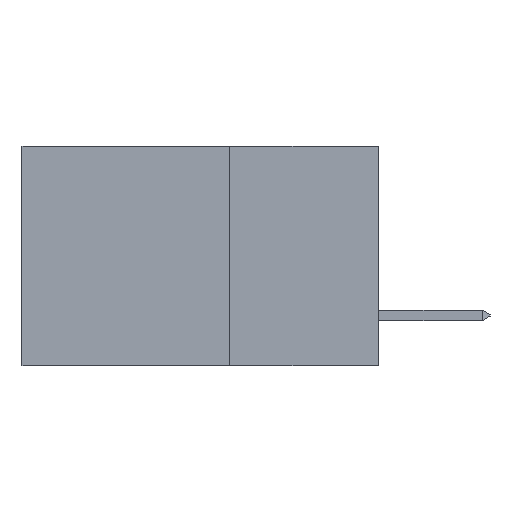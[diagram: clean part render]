
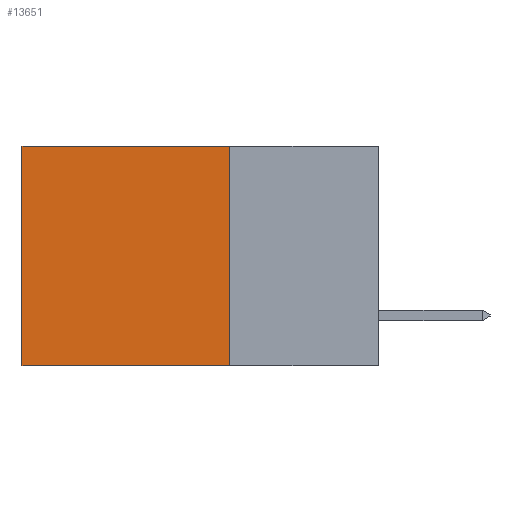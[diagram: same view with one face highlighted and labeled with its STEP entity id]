
A CAD part, left-side view. The second image highlights one B-rep face of the part: STEP entity #13651.
In plain terms, the highlighted planar face has unit normal (-1, 0, 0).
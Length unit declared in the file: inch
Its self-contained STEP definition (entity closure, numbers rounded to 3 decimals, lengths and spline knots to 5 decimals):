
#525 = CARTESIAN_POINT ( 'NONE',  ( 0.2615, 0.25, -0.37 ) ) ;
#1938 = ORIENTED_EDGE ( 'NONE', *, *, #6927, .T. ) ;
#1956 = CARTESIAN_POINT ( 'NONE',  ( 0.2615, 0.25, 0. ) ) ;
#1974 = DIRECTION ( 'NONE',  ( 0., 1., 0. ) ) ;
#3154 = LINE ( 'NONE', #15125, #6392 ) ;
#3291 = LINE ( 'NONE', #1956, #6525 ) ;
#3345 = CARTESIAN_POINT ( 'NONE',  ( 0.2615, 0.25, -0.37 ) ) ;
#3747 = LINE ( 'NONE', #525, #9693 ) ;
#4976 = EDGE_CURVE ( 'NONE', #13965, #11299, #3154, .T. ) ;
#5054 = AXIS2_PLACEMENT_3D ( 'NONE', #5770, #6984, #14944 ) ;
#5337 = ORIENTED_EDGE ( 'NONE', *, *, #14723, .F. ) ;
#5770 = CARTESIAN_POINT ( 'NONE',  ( 0.2615, 0.25, -0.37 ) ) ;
#6026 = VERTEX_POINT ( 'NONE', #8176 ) ;
#6105 = ORIENTED_EDGE ( 'NONE', *, *, #4976, .F. ) ;
#6122 = LINE ( 'NONE', #14303, #14561 ) ;
#6392 = VECTOR ( 'NONE', #14929, 39.37008 ) ;
#6525 = VECTOR ( 'NONE', #1974, 39.37008 ) ;
#6927 = EDGE_CURVE ( 'NONE', #13965, #12828, #3291, .T. ) ;
#6984 = DIRECTION ( 'NONE',  ( 1., 0., 0. ) ) ;
#7559 = CARTESIAN_POINT ( 'NONE',  ( 0.2615, 0.25, 0. ) ) ;
#8054 = EDGE_CURVE ( 'NONE', #12828, #6026, #6122, .T. ) ;
#8176 = CARTESIAN_POINT ( 'NONE',  ( 0.2615, 0.6, -0.37 ) ) ;
#9284 = PLANE ( 'NONE',  #5054 ) ;
#9693 = VECTOR ( 'NONE', #10117, 39.37008 ) ;
#10117 = DIRECTION ( 'NONE',  ( 0., 1., 0. ) ) ;
#10273 = FACE_OUTER_BOUND ( 'NONE', #11378, .T. ) ;
#11299 = VERTEX_POINT ( 'NONE', #3345 ) ;
#11378 = EDGE_LOOP ( 'NONE', ( #13143, #5337, #6105, #1938 ) ) ;
#12382 = CARTESIAN_POINT ( 'NONE',  ( 0.2615, 0.6, 0. ) ) ;
#12828 = VERTEX_POINT ( 'NONE', #12382 ) ;
#13143 = ORIENTED_EDGE ( 'NONE', *, *, #8054, .T. ) ;
#13651 = ADVANCED_FACE ( 'NONE', ( #10273 ), #9284, .F. ) ;
#13659 = DIRECTION ( 'NONE',  ( 0., 0., -1. ) ) ;
#13965 = VERTEX_POINT ( 'NONE', #7559 ) ;
#14303 = CARTESIAN_POINT ( 'NONE',  ( 0.2615, 0.6, -0.37 ) ) ;
#14561 = VECTOR ( 'NONE', #13659, 39.37008 ) ;
#14723 = EDGE_CURVE ( 'NONE', #11299, #6026, #3747, .T. ) ;
#14929 = DIRECTION ( 'NONE',  ( 0., 0., -1. ) ) ;
#14944 = DIRECTION ( 'NONE',  ( 0., 0., -1. ) ) ;
#15125 = CARTESIAN_POINT ( 'NONE',  ( 0.2615, 0.25, -0.37 ) ) ;
